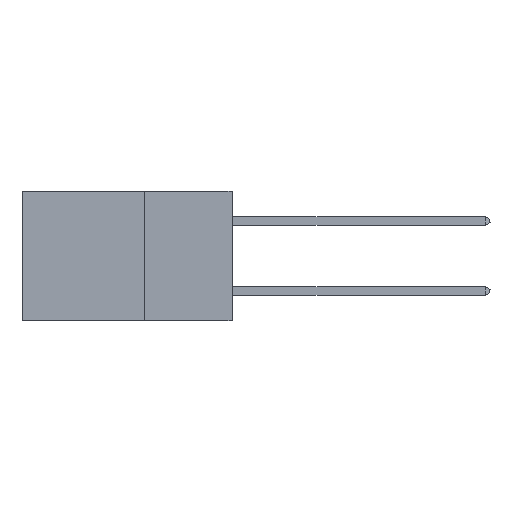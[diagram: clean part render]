
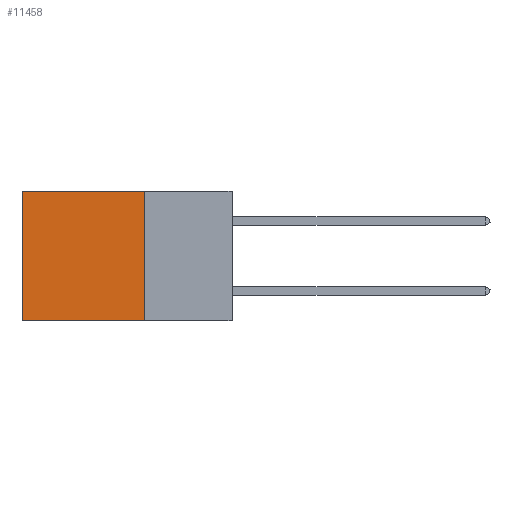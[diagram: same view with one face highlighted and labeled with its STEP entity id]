
A CAD part, left-side view. The second image highlights one B-rep face of the part: STEP entity #11458.
In plain terms, the highlighted planar face has unit normal (-1, 0, 0).
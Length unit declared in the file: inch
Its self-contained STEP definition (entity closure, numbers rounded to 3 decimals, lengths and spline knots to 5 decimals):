
#1981 = CARTESIAN_POINT ( 'NONE',  ( 0.2875, 0.6, 0. ) ) ;
#2604 = CARTESIAN_POINT ( 'NONE',  ( 0.2875, 0.25, 0. ) ) ;
#2949 = CARTESIAN_POINT ( 'NONE',  ( 0.2875, 0.25, 0. ) ) ;
#4636 = DIRECTION ( 'NONE',  ( 0., 0., -1. ) ) ;
#5047 = LINE ( 'NONE', #2604, #35480 ) ;
#6341 = LINE ( 'NONE', #2949, #27108 ) ;
#7679 = LINE ( 'NONE', #11700, #20154 ) ;
#7972 = EDGE_CURVE ( 'NONE', #27655, #24221, #7679, .T. ) ;
#11458 = ADVANCED_FACE ( 'NONE', ( #11535 ), #13452, .F. ) ;
#11535 = FACE_OUTER_BOUND ( 'NONE', #16213, .T. ) ;
#11700 = CARTESIAN_POINT ( 'NONE',  ( 0.2875, 0.6, 0. ) ) ;
#12699 = CARTESIAN_POINT ( 'NONE',  ( 0.2875, 0.25, -0.37 ) ) ;
#13439 = VERTEX_POINT ( 'NONE', #13698 ) ;
#13452 = PLANE ( 'NONE',  #35054 ) ;
#13698 = CARTESIAN_POINT ( 'NONE',  ( 0.2875, 0.25, -0.37 ) ) ;
#15248 = DIRECTION ( 'NONE',  ( 0., 1., 0. ) ) ;
#16213 = EDGE_LOOP ( 'NONE', ( #38175, #34753, #17068, #20453 ) ) ;
#16991 = DIRECTION ( 'NONE',  ( 0., 0., -1. ) ) ;
#17068 = ORIENTED_EDGE ( 'NONE', *, *, #32036, .F. ) ;
#17580 = EDGE_CURVE ( 'NONE', #23873, #27655, #6341, .T. ) ;
#19568 = DIRECTION ( 'NONE',  ( 1., 0., 0. ) ) ;
#20154 = VECTOR ( 'NONE', #16991, 39.37008 ) ;
#20453 = ORIENTED_EDGE ( 'NONE', *, *, #17580, .T. ) ;
#20938 = LINE ( 'NONE', #12699, #34319 ) ;
#22034 = CARTESIAN_POINT ( 'NONE',  ( 0.2875, 0.25, 0. ) ) ;
#22876 = DIRECTION ( 'NONE',  ( 0., 0., -1. ) ) ;
#23873 = VERTEX_POINT ( 'NONE', #22034 ) ;
#24221 = VERTEX_POINT ( 'NONE', #32437 ) ;
#27108 = VECTOR ( 'NONE', #36715, 39.37008 ) ;
#27655 = VERTEX_POINT ( 'NONE', #1981 ) ;
#28462 = CARTESIAN_POINT ( 'NONE',  ( 0.2875, 0.25, 0. ) ) ;
#29735 = EDGE_CURVE ( 'NONE', #13439, #24221, #20938, .T. ) ;
#32036 = EDGE_CURVE ( 'NONE', #23873, #13439, #5047, .T. ) ;
#32437 = CARTESIAN_POINT ( 'NONE',  ( 0.2875, 0.6, -0.37 ) ) ;
#34319 = VECTOR ( 'NONE', #15248, 39.37008 ) ;
#34753 = ORIENTED_EDGE ( 'NONE', *, *, #29735, .F. ) ;
#35054 = AXIS2_PLACEMENT_3D ( 'NONE', #28462, #19568, #4636 ) ;
#35480 = VECTOR ( 'NONE', #22876, 39.37008 ) ;
#36715 = DIRECTION ( 'NONE',  ( 0., 1., 0. ) ) ;
#38175 = ORIENTED_EDGE ( 'NONE', *, *, #7972, .T. ) ;
